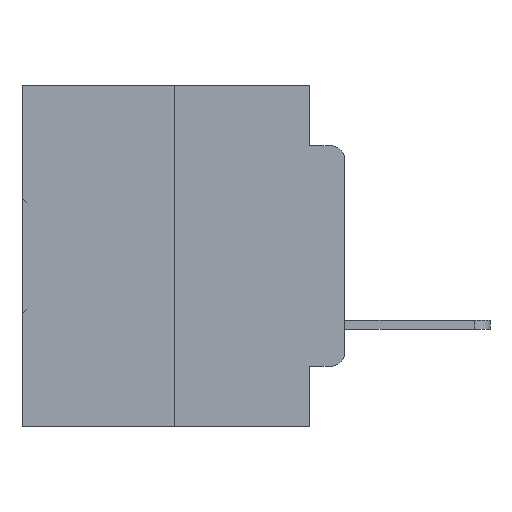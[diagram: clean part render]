
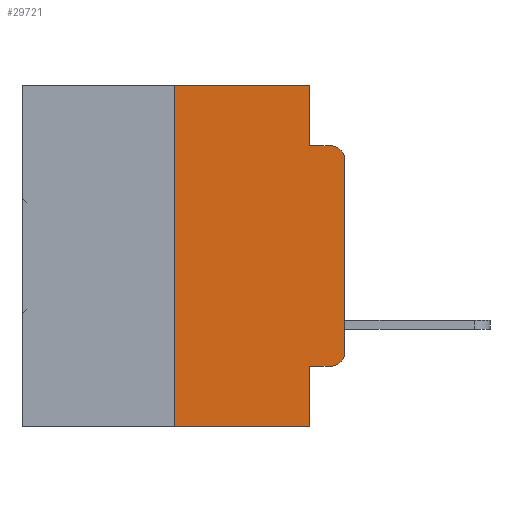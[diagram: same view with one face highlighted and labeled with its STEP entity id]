
A CAD part, left-side view. The second image highlights one B-rep face of the part: STEP entity #29721.
In plain terms, the highlighted planar face has unit normal (-1, 0, 0).
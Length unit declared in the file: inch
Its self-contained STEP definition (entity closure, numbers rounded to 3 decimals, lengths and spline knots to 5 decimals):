
#894 = EDGE_CURVE ( 'NONE', #28107, #33330, #27484, .T. ) ;
#3164 = DIRECTION ( 'NONE',  ( 0., 0., -1. ) ) ;
#4330 = LINE ( 'NONE', #19440, #34641 ) ;
#4924 = LINE ( 'NONE', #18499, #25774 ) ;
#5850 = VECTOR ( 'NONE', #33999, 39.37008 ) ;
#5985 = ORIENTED_EDGE ( 'NONE', *, *, #19374, .T. ) ;
#6017 = ORIENTED_EDGE ( 'NONE', *, *, #17531, .T. ) ;
#6433 = ORIENTED_EDGE ( 'NONE', *, *, #10169, .F. ) ;
#6491 = EDGE_CURVE ( 'NONE', #26480, #14551, #21099, .T. ) ;
#6626 = VECTOR ( 'NONE', #14824, 39.37008 ) ;
#6794 = DIRECTION ( 'NONE',  ( -1., 0., 0. ) ) ;
#7334 = ORIENTED_EDGE ( 'NONE', *, *, #8332, .F. ) ;
#7909 = ORIENTED_EDGE ( 'NONE', *, *, #9748, .F. ) ;
#8332 = EDGE_CURVE ( 'NONE', #27005, #28892, #19338, .T. ) ;
#8612 = ORIENTED_EDGE ( 'NONE', *, *, #6491, .F. ) ;
#9050 = ORIENTED_EDGE ( 'NONE', *, *, #19809, .T. ) ;
#9107 = CARTESIAN_POINT ( 'NONE',  ( 0., 0.02, -0.1085 ) ) ;
#9145 = ORIENTED_EDGE ( 'NONE', *, *, #894, .F. ) ;
#9430 = CARTESIAN_POINT ( 'NONE',  ( 0., 0., -0.3915 ) ) ;
#9541 = CARTESIAN_POINT ( 'NONE',  ( 0., 0.473, -0.5 ) ) ;
#9600 = CARTESIAN_POINT ( 'NONE',  ( 0., 0.051, -0.4115 ) ) ;
#9748 = EDGE_CURVE ( 'NONE', #14551, #27005, #4924, .T. ) ;
#10169 = EDGE_CURVE ( 'NONE', #28892, #14260, #28203, .T. ) ;
#10199 = LINE ( 'NONE', #9541, #30818 ) ;
#10240 = VECTOR ( 'NONE', #15825, 39.37008 ) ;
#10722 = VERTEX_POINT ( 'NONE', #9430 ) ;
#10749 = ORIENTED_EDGE ( 'NONE', *, *, #34137, .T. ) ;
#11191 = ORIENTED_EDGE ( 'NONE', *, *, #30653, .T. ) ;
#11786 = CARTESIAN_POINT ( 'NONE',  ( 0., 0.25, 0. ) ) ;
#11855 = DIRECTION ( 'NONE',  ( 0., 0., -1. ) ) ;
#12064 = CARTESIAN_POINT ( 'NONE',  ( 0., 0.051, -0.0885 ) ) ;
#12278 = DIRECTION ( 'NONE',  ( 0., -1., 0. ) ) ;
#13009 = VECTOR ( 'NONE', #16579, 39.37008 ) ;
#13488 = CIRCLE ( 'NONE', #17912, 0.02 ) ;
#14120 = CARTESIAN_POINT ( 'NONE',  ( 0., 0.473, 0. ) ) ;
#14260 = VERTEX_POINT ( 'NONE', #18681 ) ;
#14551 = VERTEX_POINT ( 'NONE', #11786 ) ;
#14824 = DIRECTION ( 'NONE',  ( 0., -1., 0. ) ) ;
#15825 = DIRECTION ( 'NONE',  ( 0., 0., 1. ) ) ;
#15972 = VERTEX_POINT ( 'NONE', #17205 ) ;
#16394 = AXIS2_PLACEMENT_3D ( 'NONE', #23099, #6794, #25786 ) ;
#16579 = DIRECTION ( 'NONE',  ( 0., 0., 1. ) ) ;
#16796 = CARTESIAN_POINT ( 'NONE',  ( 0., 0.25, -0.5 ) ) ;
#17205 = CARTESIAN_POINT ( 'NONE',  ( 0., 0., -0.1085 ) ) ;
#17230 = EDGE_LOOP ( 'NONE', ( #5985, #6017, #6433, #7334, #7909, #8612, #9050, #9145, #10749, #11191 ) ) ;
#17531 = EDGE_CURVE ( 'NONE', #15972, #14260, #13488, .T. ) ;
#17912 = AXIS2_PLACEMENT_3D ( 'NONE', #9107, #28006, #11855 ) ;
#18069 = CARTESIAN_POINT ( 'NONE',  ( 0., 0.051, 0. ) ) ;
#18123 = VERTEX_POINT ( 'NONE', #22649 ) ;
#18499 = CARTESIAN_POINT ( 'NONE',  ( 0., 0.473, 0. ) ) ;
#18681 = CARTESIAN_POINT ( 'NONE',  ( 0., 0.02, -0.0885 ) ) ;
#19338 = LINE ( 'NONE', #24906, #33350 ) ;
#19374 = EDGE_CURVE ( 'NONE', #10722, #15972, #31663, .T. ) ;
#19440 = CARTESIAN_POINT ( 'NONE',  ( 0., 0.051, -0.4115 ) ) ;
#19605 = FACE_OUTER_BOUND ( 'NONE', #17230, .T. ) ;
#19654 = DIRECTION ( 'NONE',  ( 1., 0., 0. ) ) ;
#19809 = EDGE_CURVE ( 'NONE', #26480, #33330, #10199, .T. ) ;
#21099 = LINE ( 'NONE', #29852, #13009 ) ;
#22099 = DIRECTION ( 'NONE',  ( 0., -1., 0. ) ) ;
#22649 = CARTESIAN_POINT ( 'NONE',  ( 0., 0.02, -0.4115 ) ) ;
#23099 = CARTESIAN_POINT ( 'NONE',  ( 0., 0.02, -0.3915 ) ) ;
#24880 = PLANE ( 'NONE',  #34983 ) ;
#24906 = CARTESIAN_POINT ( 'NONE',  ( 0., 0.051, 0. ) ) ;
#25774 = VECTOR ( 'NONE', #31702, 39.37008 ) ;
#25786 = DIRECTION ( 'NONE',  ( 0., 0., -1. ) ) ;
#26480 = VERTEX_POINT ( 'NONE', #16796 ) ;
#26719 = CARTESIAN_POINT ( 'NONE',  ( 0., 0.051, -0.0885 ) ) ;
#26959 = CARTESIAN_POINT ( 'NONE',  ( 0., 0.051, 0. ) ) ;
#27005 = VERTEX_POINT ( 'NONE', #26959 ) ;
#27484 = LINE ( 'NONE', #18069, #5850 ) ;
#27572 = DIRECTION ( 'NONE',  ( 0., 0., -1. ) ) ;
#28006 = DIRECTION ( 'NONE',  ( -1., 0., 0. ) ) ;
#28107 = VERTEX_POINT ( 'NONE', #9600 ) ;
#28203 = LINE ( 'NONE', #12064, #6626 ) ;
#28892 = VERTEX_POINT ( 'NONE', #26719 ) ;
#29721 = ADVANCED_FACE ( 'NONE', ( #19605 ), #24880, .F. ) ;
#29852 = CARTESIAN_POINT ( 'NONE',  ( 0., 0.25, 0. ) ) ;
#30459 = CIRCLE ( 'NONE', #16394, 0.02 ) ;
#30653 = EDGE_CURVE ( 'NONE', #18123, #10722, #30459, .T. ) ;
#30818 = VECTOR ( 'NONE', #12278, 39.37008 ) ;
#31663 = LINE ( 'NONE', #34373, #10240 ) ;
#31702 = DIRECTION ( 'NONE',  ( 0., -1., 0. ) ) ;
#31750 = CARTESIAN_POINT ( 'NONE',  ( 0., 0.051, -0.5 ) ) ;
#33330 = VERTEX_POINT ( 'NONE', #31750 ) ;
#33350 = VECTOR ( 'NONE', #27572, 39.37008 ) ;
#33999 = DIRECTION ( 'NONE',  ( 0., 0., -1. ) ) ;
#34137 = EDGE_CURVE ( 'NONE', #28107, #18123, #4330, .T. ) ;
#34373 = CARTESIAN_POINT ( 'NONE',  ( 0., 0., 0. ) ) ;
#34641 = VECTOR ( 'NONE', #22099, 39.37008 ) ;
#34983 = AXIS2_PLACEMENT_3D ( 'NONE', #14120, #19654, #3164 ) ;
